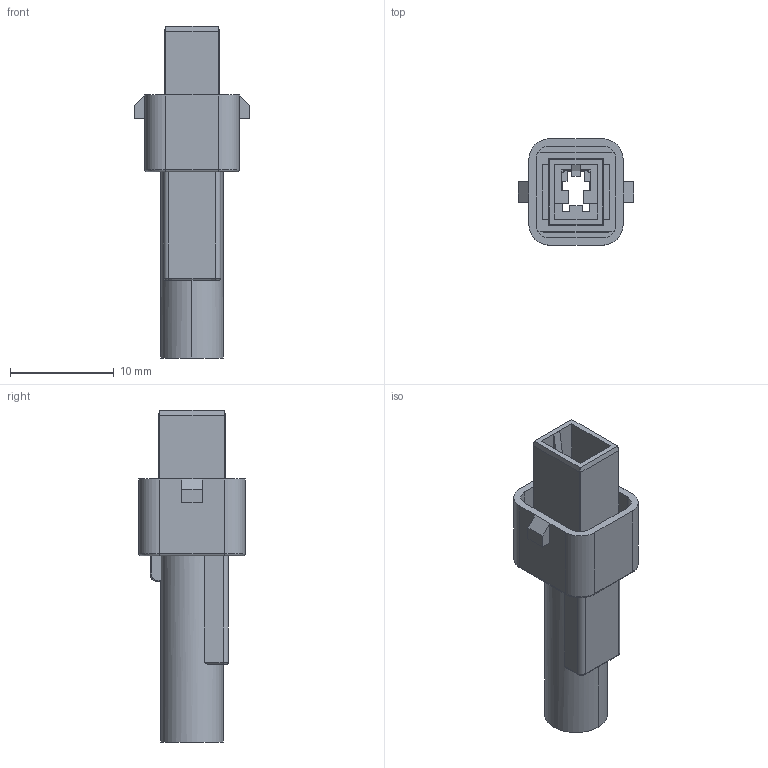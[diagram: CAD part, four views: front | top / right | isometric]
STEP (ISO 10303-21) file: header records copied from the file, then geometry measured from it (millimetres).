
FILE_DESCRIPTION (( 'STEP AP214' ), '1' );
FILE_NAME ('568-001-000-100.STEP', '2020-07-29T15:31:50', ( '' ), ( '' ), 'SwSTEP 2.0', 'SolidWorks 2020', '' );
FILE_SCHEMA (( 'AUTOMOTIVE_DESIGN' ));
Length unit declared in the file: millimetre
Products named in the file (3): 568-001-000-100_Silicon Rubber; 568-001-000-100; 568-001-000-100_Housing
Assembly tree (2 placements, depth 2):
  568-001-000-100
    568-001-000-100_Housing
    568-001-000-100_Silicon Rubber
Bounding box: 11.1 x 10.25 x 32 mm (x, y, z)
Volume: 768.1 mm3; surface area: 2075.4 mm2
Topology: 2 solids, 2 shells, 176 faces, 448 edges, 283 vertices
Faces by surface type: plane 101, cylinder 47, torus 14, bspline 10, cone 4
Entity records: 5556 total; most frequent: CARTESIAN_POINT 1227, ORIENTED_EDGE 896, DIRECTION 871, EDGE_CURVE 448, LINE 291, VECTOR 291, AXIS2_PLACEMENT_3D 290, VERTEX_POINT 283
